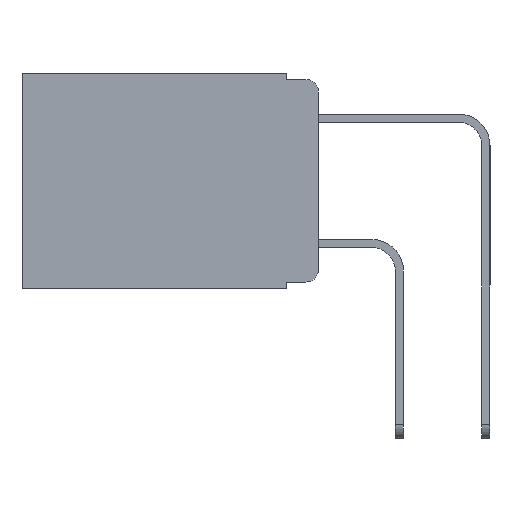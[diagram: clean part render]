
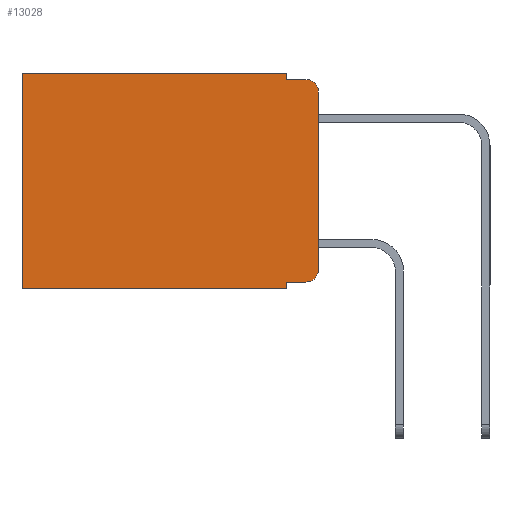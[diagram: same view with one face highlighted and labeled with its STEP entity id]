
A CAD part, left-side view. The second image highlights one B-rep face of the part: STEP entity #13028.
In plain terms, the highlighted planar face has unit normal (-1, 0, 0).
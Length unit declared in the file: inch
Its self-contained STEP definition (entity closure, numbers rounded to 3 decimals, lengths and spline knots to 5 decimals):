
#311 = EDGE_CURVE ( 'NONE', #4629, #9526, #4664, .T. ) ;
#475 = CARTESIAN_POINT ( 'NONE',  ( 0.298, 0.02, -0.01 ) ) ;
#558 = VERTEX_POINT ( 'NONE', #727 ) ;
#727 = CARTESIAN_POINT ( 'NONE',  ( 0.298, 0.473, -0.343 ) ) ;
#909 = LINE ( 'NONE', #15315, #4483 ) ;
#1116 = VERTEX_POINT ( 'NONE', #15703 ) ;
#1432 = ORIENTED_EDGE ( 'NONE', *, *, #9054, .F. ) ;
#1459 = DIRECTION ( 'NONE',  ( 0., 0., -1. ) ) ;
#1520 = VERTEX_POINT ( 'NONE', #7508 ) ;
#1725 = VECTOR ( 'NONE', #1459, 39.37008 ) ;
#2067 = VECTOR ( 'NONE', #2256, 39.37008 ) ;
#2256 = DIRECTION ( 'NONE',  ( 0., 0., -1. ) ) ;
#3150 = VECTOR ( 'NONE', #13893, 39.37008 ) ;
#3259 = CARTESIAN_POINT ( 'NONE',  ( 0.298, 0., 0. ) ) ;
#3267 = VERTEX_POINT ( 'NONE', #5647 ) ;
#3552 = DIRECTION ( 'NONE',  ( 0., 0., -1. ) ) ;
#3968 = ORIENTED_EDGE ( 'NONE', *, *, #14393, .F. ) ;
#4327 = AXIS2_PLACEMENT_3D ( 'NONE', #8007, #8021, #6449 ) ;
#4388 = DIRECTION ( 'NONE',  ( 0., 1., 0. ) ) ;
#4428 = EDGE_CURVE ( 'NONE', #1520, #558, #9401, .T. ) ;
#4464 = VECTOR ( 'NONE', #14368, 39.37008 ) ;
#4483 = VECTOR ( 'NONE', #8270, 39.37008 ) ;
#4571 = DIRECTION ( 'NONE',  ( 0., 0., -1. ) ) ;
#4629 = VERTEX_POINT ( 'NONE', #6047 ) ;
#4664 = CIRCLE ( 'NONE', #4327, 0.02 ) ;
#4674 = CIRCLE ( 'NONE', #12605, 0.02 ) ;
#5019 = CARTESIAN_POINT ( 'NONE',  ( 0.298, 0.02, -0.313 ) ) ;
#5143 = CARTESIAN_POINT ( 'NONE',  ( 0.298, 0.051, -0.01 ) ) ;
#5647 = CARTESIAN_POINT ( 'NONE',  ( 0.298, 0.02, -0.333 ) ) ;
#5648 = LINE ( 'NONE', #10301, #1725 ) ;
#5759 = VECTOR ( 'NONE', #4388, 39.37008 ) ;
#6000 = ORIENTED_EDGE ( 'NONE', *, *, #14834, .T. ) ;
#6021 = CARTESIAN_POINT ( 'NONE',  ( 0.298, 0.051, -0.333 ) ) ;
#6047 = CARTESIAN_POINT ( 'NONE',  ( 0.298, 0., -0.03 ) ) ;
#6319 = DIRECTION ( 'NONE',  ( 0., 0., -1. ) ) ;
#6449 = DIRECTION ( 'NONE',  ( 0., 0., -1. ) ) ;
#7413 = FACE_OUTER_BOUND ( 'NONE', #15415, .T. ) ;
#7508 = CARTESIAN_POINT ( 'NONE',  ( 0.298, 0.051, -0.343 ) ) ;
#8007 = CARTESIAN_POINT ( 'NONE',  ( 0.298, 0.02, -0.03 ) ) ;
#8021 = DIRECTION ( 'NONE',  ( -1., 0., 0. ) ) ;
#8040 = CARTESIAN_POINT ( 'NONE',  ( 0.298, 0.473, 0. ) ) ;
#8258 = PLANE ( 'NONE',  #10361 ) ;
#8270 = DIRECTION ( 'NONE',  ( 0., 1., 0. ) ) ;
#8456 = CARTESIAN_POINT ( 'NONE',  ( 0.298, 0.051, 0. ) ) ;
#8722 = EDGE_CURVE ( 'NONE', #14024, #558, #15970, .T. ) ;
#9054 = EDGE_CURVE ( 'NONE', #15801, #1116, #11661, .T. ) ;
#9401 = LINE ( 'NONE', #10545, #5759 ) ;
#9526 = VERTEX_POINT ( 'NONE', #475 ) ;
#9695 = VECTOR ( 'NONE', #3552, 39.37008 ) ;
#10180 = ORIENTED_EDGE ( 'NONE', *, *, #311, .T. ) ;
#10301 = CARTESIAN_POINT ( 'NONE',  ( 0.298, 0., 0. ) ) ;
#10361 = AXIS2_PLACEMENT_3D ( 'NONE', #3259, #11895, #4571 ) ;
#10545 = CARTESIAN_POINT ( 'NONE',  ( 0.298, 0., -0.343 ) ) ;
#10958 = CARTESIAN_POINT ( 'NONE',  ( 0.298, 0., -0.313 ) ) ;
#11507 = EDGE_CURVE ( 'NONE', #15801, #14024, #909, .T. ) ;
#11661 = LINE ( 'NONE', #12208, #2067 ) ;
#11737 = EDGE_CURVE ( 'NONE', #3267, #15864, #4674, .T. ) ;
#11761 = VECTOR ( 'NONE', #13597, 39.37008 ) ;
#11828 = VERTEX_POINT ( 'NONE', #12463 ) ;
#11895 = DIRECTION ( 'NONE',  ( 1., 0., 0. ) ) ;
#11940 = ORIENTED_EDGE ( 'NONE', *, *, #4428, .F. ) ;
#12145 = CARTESIAN_POINT ( 'NONE',  ( 0.298, 0.051, 0. ) ) ;
#12208 = CARTESIAN_POINT ( 'NONE',  ( 0.298, 0.051, 0. ) ) ;
#12238 = EDGE_CURVE ( 'NONE', #11828, #1520, #12470, .T. ) ;
#12287 = ORIENTED_EDGE ( 'NONE', *, *, #11507, .T. ) ;
#12463 = CARTESIAN_POINT ( 'NONE',  ( 0.298, 0.051, -0.333 ) ) ;
#12470 = LINE ( 'NONE', #12145, #9695 ) ;
#12605 = AXIS2_PLACEMENT_3D ( 'NONE', #5019, #13489, #6319 ) ;
#12775 = CARTESIAN_POINT ( 'NONE',  ( 0.298, 0.473, 0. ) ) ;
#13028 = ADVANCED_FACE ( 'NONE', ( #7413 ), #8258, .F. ) ;
#13222 = ORIENTED_EDGE ( 'NONE', *, *, #15171, .F. ) ;
#13327 = ORIENTED_EDGE ( 'NONE', *, *, #11737, .T. ) ;
#13379 = ORIENTED_EDGE ( 'NONE', *, *, #8722, .T. ) ;
#13489 = DIRECTION ( 'NONE',  ( -1., 0., 0. ) ) ;
#13597 = DIRECTION ( 'NONE',  ( 0., -1., 0. ) ) ;
#13893 = DIRECTION ( 'NONE',  ( 0., 0., -1. ) ) ;
#14024 = VERTEX_POINT ( 'NONE', #8040 ) ;
#14098 = LINE ( 'NONE', #6021, #4464 ) ;
#14368 = DIRECTION ( 'NONE',  ( 0., -1., 0. ) ) ;
#14393 = EDGE_CURVE ( 'NONE', #1116, #9526, #14469, .T. ) ;
#14469 = LINE ( 'NONE', #5143, #11761 ) ;
#14834 = EDGE_CURVE ( 'NONE', #11828, #3267, #14098, .T. ) ;
#15144 = ORIENTED_EDGE ( 'NONE', *, *, #12238, .F. ) ;
#15171 = EDGE_CURVE ( 'NONE', #4629, #15864, #5648, .T. ) ;
#15315 = CARTESIAN_POINT ( 'NONE',  ( 0.298, 0., 0. ) ) ;
#15415 = EDGE_LOOP ( 'NONE', ( #13222, #10180, #3968, #1432, #12287, #13379, #11940, #15144, #6000, #13327 ) ) ;
#15703 = CARTESIAN_POINT ( 'NONE',  ( 0.298, 0.051, -0.01 ) ) ;
#15801 = VERTEX_POINT ( 'NONE', #8456 ) ;
#15864 = VERTEX_POINT ( 'NONE', #10958 ) ;
#15970 = LINE ( 'NONE', #12775, #3150 ) ;
